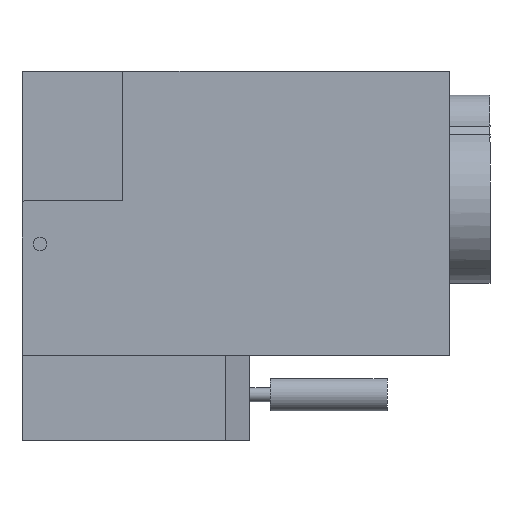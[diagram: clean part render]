
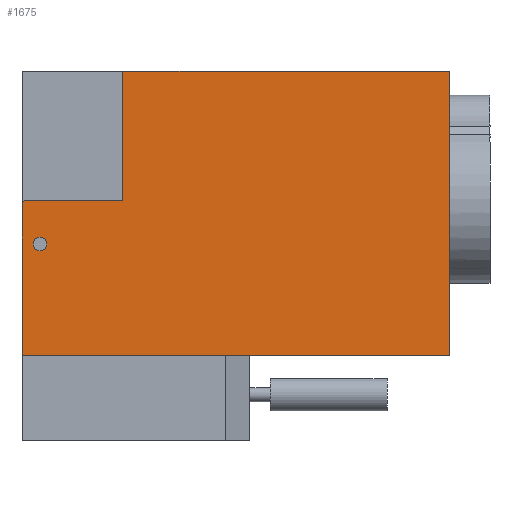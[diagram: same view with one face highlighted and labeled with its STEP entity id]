
A CAD part, left-side view. The second image highlights one B-rep face of the part: STEP entity #1675.
In plain terms, the highlighted planar face has unit normal (-1, 0, 0).
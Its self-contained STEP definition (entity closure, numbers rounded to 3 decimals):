
#53=B_SPLINE_CURVE_WITH_KNOTS('',3,(#2477,#2478,#2479,#2480),
 .UNSPECIFIED.,.F.,.F.,(4,4),(-0.986,-0.88),
 .UNSPECIFIED.);
#75=FACE_BOUND('',#247,.T.);
#84=CIRCLE('',#1756,1.65);
#153=FACE_OUTER_BOUND('',#246,.T.);
#246=EDGE_LOOP('',(#1301,#1302,#1303,#1304,#1305,#1306,#1307));
#247=EDGE_LOOP('',(#1308));
#304=LINE('',#2321,#486);
#308=LINE('',#2331,#490);
#347=LINE('',#2429,#529);
#349=LINE('',#2433,#531);
#360=LINE('',#2533,#542);
#369=LINE('',#2567,#551);
#486=VECTOR('',#1878,10.);
#490=VECTOR('',#1884,10.);
#529=VECTOR('',#1943,10.);
#531=VECTOR('',#1947,10.);
#542=VECTOR('',#1980,10.);
#551=VECTOR('',#2009,10.);
#665=VERTEX_POINT('',#2314);
#668=VERTEX_POINT('',#2319);
#672=VERTEX_POINT('',#2328);
#673=VERTEX_POINT('',#2330);
#709=VERTEX_POINT('',#2415);
#710=VERTEX_POINT('',#2428);
#711=VERTEX_POINT('',#2432);
#718=VERTEX_POINT('',#2456);
#832=EDGE_CURVE('',#668,#665,#304,.F.);
#836=EDGE_CURVE('',#673,#672,#308,.T.);
#879=EDGE_CURVE('',#710,#709,#347,.F.);
#881=EDGE_CURVE('',#673,#711,#349,.F.);
#889=EDGE_CURVE('',#718,#718,#84,.F.);
#892=EDGE_CURVE('',#709,#711,#53,.T.);
#904=EDGE_CURVE('',#710,#668,#360,.F.);
#920=EDGE_CURVE('',#665,#672,#369,.F.);
#1301=ORIENTED_EDGE('',*,*,#836,.T.);
#1302=ORIENTED_EDGE('',*,*,#920,.F.);
#1303=ORIENTED_EDGE('',*,*,#832,.F.);
#1304=ORIENTED_EDGE('',*,*,#904,.F.);
#1305=ORIENTED_EDGE('',*,*,#879,.T.);
#1306=ORIENTED_EDGE('',*,*,#892,.T.);
#1307=ORIENTED_EDGE('',*,*,#881,.F.);
#1308=ORIENTED_EDGE('',*,*,#889,.T.);
#1597=PLANE('',#1797);
#1675=ADVANCED_FACE('',(#153,#75),#1597,.F.);
#1756=AXIS2_PLACEMENT_3D('',#2457,#1957,#1958);
#1797=AXIS2_PLACEMENT_3D('',#2701,#2075,#2076);
#1878=DIRECTION('',(0.,1.,0.));
#1884=DIRECTION('',(0.,-1.,0.));
#1943=DIRECTION('',(0.,-1.,0.));
#1947=DIRECTION('',(0.,0.,-1.));
#1957=DIRECTION('center_axis',(-1.,0.,0.));
#1958=DIRECTION('ref_axis',(0.,-1.,0.));
#1980=DIRECTION('',(0.,0.,-1.));
#2009=DIRECTION('',(0.,0.,1.));
#2075=DIRECTION('center_axis',(1.,0.,0.));
#2076=DIRECTION('ref_axis',(0.,0.,-1.));
#2314=CARTESIAN_POINT('',(-28.,-64.389,20.409));
#2319=CARTESIAN_POINT('',(-28.,16.611,20.409));
#2321=CARTESIAN_POINT('',(-28.,-46.121,20.409));
#2328=CARTESIAN_POINT('',(-28.,-64.389,-50.08));
#2330=CARTESIAN_POINT('',(-28.,41.611,-50.08));
#2331=CARTESIAN_POINT('',(-28.,-84.771,-50.08));
#2415=CARTESIAN_POINT('',(-28.,41.026,-11.571));
#2428=CARTESIAN_POINT('',(-28.,16.611,-11.571));
#2429=CARTESIAN_POINT('',(-28.,-19.216,-11.571));
#2432=CARTESIAN_POINT('',(-28.,41.611,-12.443));
#2433=CARTESIAN_POINT('',(-28.,41.611,-20.163));
#2456=CARTESIAN_POINT('',(-28.,38.787,-22.384));
#2457=CARTESIAN_POINT('Origin',(-28.,37.137,-22.384));
#2477=CARTESIAN_POINT('Ctrl Pts',(-28.,41.026,-11.571));
#2478=CARTESIAN_POINT('Ctrl Pts',(-28.,41.205,-11.872));
#2479=CARTESIAN_POINT('Ctrl Pts',(-28.,41.401,-12.163));
#2480=CARTESIAN_POINT('Ctrl Pts',(-28.,41.611,-12.443));
#2533=CARTESIAN_POINT('',(-28.,16.611,-13.461));
#2567=CARTESIAN_POINT('',(-28.,-64.389,-12.248));
#2701=CARTESIAN_POINT('Origin',(-28.,-56.412,-12.003));
